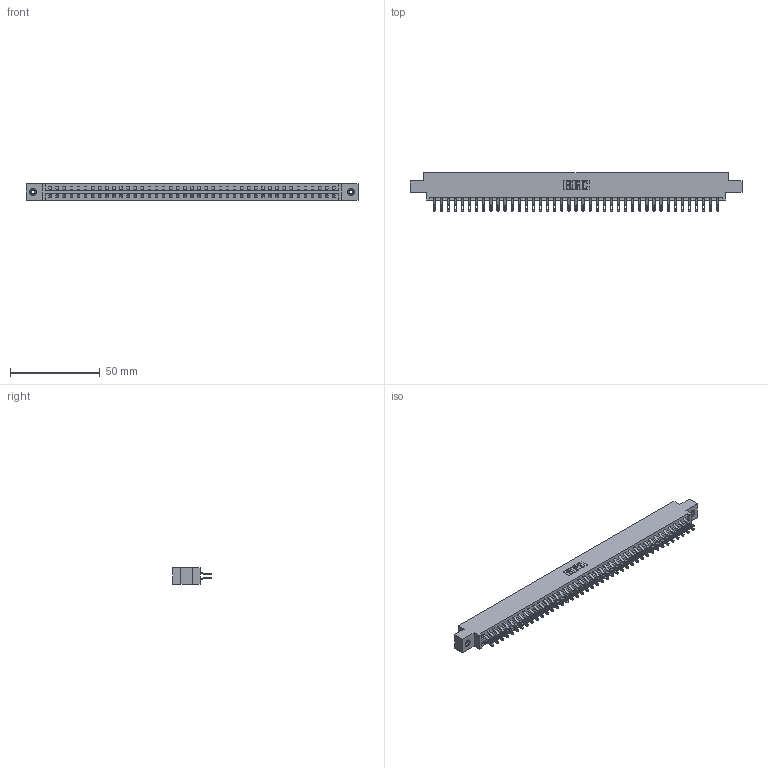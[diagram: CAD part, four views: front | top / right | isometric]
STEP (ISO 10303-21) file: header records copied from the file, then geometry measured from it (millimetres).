
FILE_DESCRIPTION (( 'STEP AP203' ), '1' );
FILE_NAME ('387-082-555-808.STEP', '2018-09-23T20:42:34', ( '' ), ( '' ), 'SwSTEP 2.0', 'SolidWorks 2016', '' );
FILE_SCHEMA (( 'CONFIG_CONTROL_DESIGN' ));
Length unit declared in the file: inch
Products named in the file (4): 337 Part_0.170 Offset - 0.156 Dia-TI; 345-292-001_555 Tail; 345-250-001_345-250-003-102; 387-082-555-808
Assembly tree (85 placements, depth 2):
  387-082-555-808
    337 Part_0.170 Offset - 0.156 Dia-TI
    345-292-001_555 Tail  x82
    345-250-001_345-250-003-102  x2
Bounding box: 185.47 x 21.47 x 9.4 mm (x, y, z)
Volume: 19646.9 mm3; surface area: 23229.2 mm2
Topology: 85 solids, 85 shells, 5098 faces, 15957 edges, 10630 vertices
Faces by surface type: plane 3058, cylinder 2024, cone 12, torus 4
Entity records: 33562 total; most frequent: CARTESIAN_POINT 5671, ORIENTED_EDGE 5570, DIRECTION 4827, EDGE_CURVE 2785, LINE 2617, VECTOR 2617, VERTEX_POINT 1852, AXIS2_PLACEMENT_3D 1105
